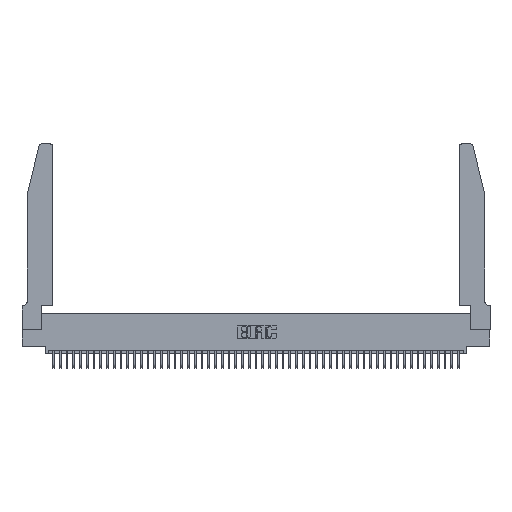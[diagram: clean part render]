
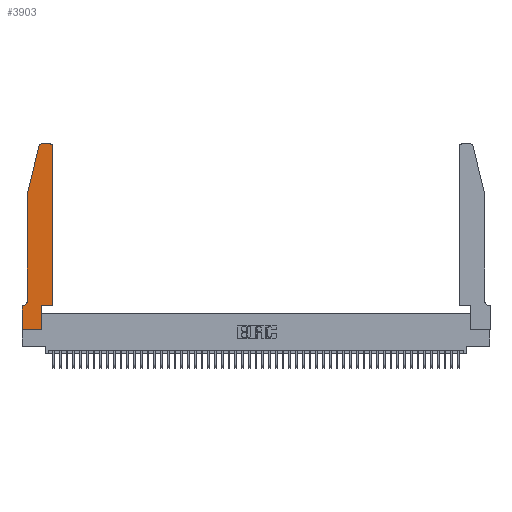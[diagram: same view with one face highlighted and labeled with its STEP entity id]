
A CAD part, top view. The second image highlights one B-rep face of the part: STEP entity #3903.
In plain terms, the highlighted planar face has unit normal (0, 0, 1).
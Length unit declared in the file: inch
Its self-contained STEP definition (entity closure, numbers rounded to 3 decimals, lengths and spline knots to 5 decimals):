
#424 = DIRECTION ( 'NONE',  ( -1., 0., 0. ) ) ;
#1851 = CARTESIAN_POINT ( 'NONE',  ( 0.2605, 2.75, 0.37 ) ) ;
#2038 = CARTESIAN_POINT ( 'NONE',  ( 0., 0.35, 0.37 ) ) ;
#2261 = DIRECTION ( 'NONE',  ( 1., 0., 0. ) ) ;
#2665 = LINE ( 'NONE', #24000, #35338 ) ;
#3143 = EDGE_CURVE ( 'NONE', #40586, #39088, #6658, .T. ) ;
#3330 = LINE ( 'NONE', #11355, #3941 ) ;
#3443 = DIRECTION ( 'NONE',  ( 0., 1., 0. ) ) ;
#3717 = CARTESIAN_POINT ( 'NONE',  ( 0.4505, 0.35, 0.37 ) ) ;
#3903 = ADVANCED_FACE ( 'NONE', ( #19112 ), #45104, .T. ) ;
#3941 = VECTOR ( 'NONE', #3443, 39.37008 ) ;
#4476 = EDGE_CURVE ( 'NONE', #40450, #28640, #2665, .T. ) ;
#5321 = AXIS2_PLACEMENT_3D ( 'NONE', #8224, #39936, #40460 ) ;
#6658 = LINE ( 'NONE', #25210, #46753 ) ;
#7156 = ORIENTED_EDGE ( 'NONE', *, *, #48802, .T. ) ;
#7496 = CARTESIAN_POINT ( 'NONE',  ( 0.2865, 0.35, 0.37 ) ) ;
#8131 = CARTESIAN_POINT ( 'NONE',  ( 0., 0., 0.37 ) ) ;
#8224 = CARTESIAN_POINT ( 'NONE',  ( 0.4205, 2.72, 0.37 ) ) ;
#9133 = ORIENTED_EDGE ( 'NONE', *, *, #30874, .T. ) ;
#10867 = CARTESIAN_POINT ( 'NONE',  ( 0.4505, 2.72, 0.37 ) ) ;
#11273 = VERTEX_POINT ( 'NONE', #50116 ) ;
#11355 = CARTESIAN_POINT ( 'NONE',  ( 0.2865, 0.35, 0.37 ) ) ;
#12708 = DIRECTION ( 'NONE',  ( 1., 0., 0. ) ) ;
#14052 = ORIENTED_EDGE ( 'NONE', *, *, #24252, .T. ) ;
#14350 = VERTEX_POINT ( 'NONE', #30318 ) ;
#14570 = VERTEX_POINT ( 'NONE', #32397 ) ;
#15937 = VECTOR ( 'NONE', #31503, 39.37008 ) ;
#16458 = EDGE_CURVE ( 'NONE', #28640, #36986, #48936, .T. ) ;
#17401 = ORIENTED_EDGE ( 'NONE', *, *, #35416, .T. ) ;
#18769 = ORIENTED_EDGE ( 'NONE', *, *, #47822, .T. ) ;
#19112 = FACE_OUTER_BOUND ( 'NONE', #30654, .T. ) ;
#19644 = CIRCLE ( 'NONE', #30076, 0.03 ) ;
#20017 = CARTESIAN_POINT ( 'NONE',  ( 0.0055, 0.35, 0.37 ) ) ;
#20018 = AXIS2_PLACEMENT_3D ( 'NONE', #28790, #44936, #12708 ) ;
#20870 = LINE ( 'NONE', #1851, #24640 ) ;
#20949 = DIRECTION ( 'NONE',  ( 1., 0., 0. ) ) ;
#20994 = ORIENTED_EDGE ( 'NONE', *, *, #3143, .T. ) ;
#24000 = CARTESIAN_POINT ( 'NONE',  ( 0.4505, 0.35, 0.37 ) ) ;
#24252 = EDGE_CURVE ( 'NONE', #14350, #33687, #38527, .T. ) ;
#24586 = DIRECTION ( 'NONE',  ( 1., 0., 0. ) ) ;
#24640 = VECTOR ( 'NONE', #37445, 39.37008 ) ;
#25210 = CARTESIAN_POINT ( 'NONE',  ( 0.0755, 0.35, 0.37 ) ) ;
#25258 = VERTEX_POINT ( 'NONE', #49604 ) ;
#25305 = DIRECTION ( 'NONE',  ( 0., 0., 1. ) ) ;
#26085 = ORIENTED_EDGE ( 'NONE', *, *, #26850, .T. ) ;
#26496 = ORIENTED_EDGE ( 'NONE', *, *, #28704, .T. ) ;
#26850 = EDGE_CURVE ( 'NONE', #11273, #25258, #37888, .T. ) ;
#28206 = CARTESIAN_POINT ( 'NONE',  ( 0., 0., 0.37 ) ) ;
#28309 = CARTESIAN_POINT ( 'NONE',  ( 0.0755, 2., 0.37 ) ) ;
#28388 = DIRECTION ( 'NONE',  ( 0., -1., 0. ) ) ;
#28640 = VERTEX_POINT ( 'NONE', #10867 ) ;
#28704 = EDGE_CURVE ( 'NONE', #36947, #40450, #31772, .T. ) ;
#28790 = CARTESIAN_POINT ( 'NONE',  ( 0., 0.35, 0.37 ) ) ;
#28874 = ORIENTED_EDGE ( 'NONE', *, *, #16458, .T. ) ;
#28893 = DIRECTION ( 'NONE',  ( -1., 0., 0. ) ) ;
#29393 = VECTOR ( 'NONE', #33255, 39.37008 ) ;
#29952 = VERTEX_POINT ( 'NONE', #49976 ) ;
#30076 = AXIS2_PLACEMENT_3D ( 'NONE', #37073, #25305, #20949 ) ;
#30318 = CARTESIAN_POINT ( 'NONE',  ( 0.0755, 2., 0.37 ) ) ;
#30654 = EDGE_LOOP ( 'NONE', ( #18769, #9133, #46502, #14052, #36001, #20994, #7156, #26085, #17401, #26496, #45975, #28874 ) ) ;
#30874 = EDGE_CURVE ( 'NONE', #14570, #29952, #19644, .T. ) ;
#30877 = CIRCLE ( 'NONE', #32233, 0.07 ) ;
#31503 = DIRECTION ( 'NONE',  ( 0., -1., 0. ) ) ;
#31772 = LINE ( 'NONE', #46926, #46196 ) ;
#32233 = AXIS2_PLACEMENT_3D ( 'NONE', #47862, #35999, #424 ) ;
#32397 = CARTESIAN_POINT ( 'NONE',  ( 0.284, 2.75, 0.37 ) ) ;
#32889 = CARTESIAN_POINT ( 'NONE',  ( 0.0755, 0.42, 0.37 ) ) ;
#33255 = DIRECTION ( 'NONE',  ( -0.239, -0.971, 0. ) ) ;
#33687 = VERTEX_POINT ( 'NONE', #32889 ) ;
#35338 = VECTOR ( 'NONE', #44700, 39.37008 ) ;
#35416 = EDGE_CURVE ( 'NONE', #25258, #36947, #3330, .T. ) ;
#35999 = DIRECTION ( 'NONE',  ( 0., 0., -1. ) ) ;
#36001 = ORIENTED_EDGE ( 'NONE', *, *, #48268, .T. ) ;
#36632 = VECTOR ( 'NONE', #24586, 39.37008 ) ;
#36892 = LINE ( 'NONE', #28309, #29393 ) ;
#36947 = VERTEX_POINT ( 'NONE', #7496 ) ;
#36986 = VERTEX_POINT ( 'NONE', #48809 ) ;
#37073 = CARTESIAN_POINT ( 'NONE',  ( 0.284, 2.72, 0.37 ) ) ;
#37445 = DIRECTION ( 'NONE',  ( -1., 0., 0. ) ) ;
#37888 = LINE ( 'NONE', #8131, #36632 ) ;
#38527 = LINE ( 'NONE', #39734, #15937 ) ;
#39088 = VERTEX_POINT ( 'NONE', #2038 ) ;
#39734 = CARTESIAN_POINT ( 'NONE',  ( 0.0755, 2., 0.37 ) ) ;
#39936 = DIRECTION ( 'NONE',  ( 0., 0., 1. ) ) ;
#40450 = VERTEX_POINT ( 'NONE', #3717 ) ;
#40460 = DIRECTION ( 'NONE',  ( 1., 0., 0. ) ) ;
#40586 = VERTEX_POINT ( 'NONE', #20017 ) ;
#44700 = DIRECTION ( 'NONE',  ( 0., 1., 0. ) ) ;
#44936 = DIRECTION ( 'NONE',  ( 0., 0., 1. ) ) ;
#45104 = PLANE ( 'NONE',  #20018 ) ;
#45272 = LINE ( 'NONE', #28206, #48944 ) ;
#45975 = ORIENTED_EDGE ( 'NONE', *, *, #4476, .T. ) ;
#46196 = VECTOR ( 'NONE', #2261, 39.37008 ) ;
#46502 = ORIENTED_EDGE ( 'NONE', *, *, #51444, .T. ) ;
#46753 = VECTOR ( 'NONE', #28893, 39.37008 ) ;
#46926 = CARTESIAN_POINT ( 'NONE',  ( 0.4505, 0.35, 0.37 ) ) ;
#47822 = EDGE_CURVE ( 'NONE', #36986, #14570, #20870, .T. ) ;
#47862 = CARTESIAN_POINT ( 'NONE',  ( 0.0055, 0.42, 0.37 ) ) ;
#48268 = EDGE_CURVE ( 'NONE', #33687, #40586, #30877, .T. ) ;
#48802 = EDGE_CURVE ( 'NONE', #39088, #11273, #45272, .T. ) ;
#48809 = CARTESIAN_POINT ( 'NONE',  ( 0.4205, 2.75, 0.37 ) ) ;
#48936 = CIRCLE ( 'NONE', #5321, 0.03 ) ;
#48944 = VECTOR ( 'NONE', #28388, 39.37008 ) ;
#49604 = CARTESIAN_POINT ( 'NONE',  ( 0.2865, 0., 0.37 ) ) ;
#49976 = CARTESIAN_POINT ( 'NONE',  ( 0.25487, 2.72718, 0.37 ) ) ;
#50116 = CARTESIAN_POINT ( 'NONE',  ( 0., 0., 0.37 ) ) ;
#51444 = EDGE_CURVE ( 'NONE', #29952, #14350, #36892, .T. ) ;
